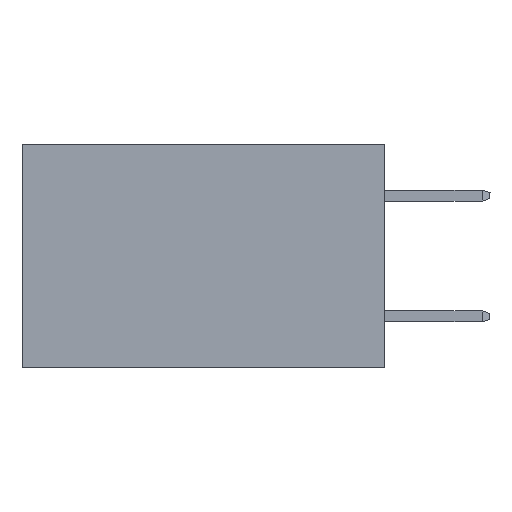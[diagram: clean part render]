
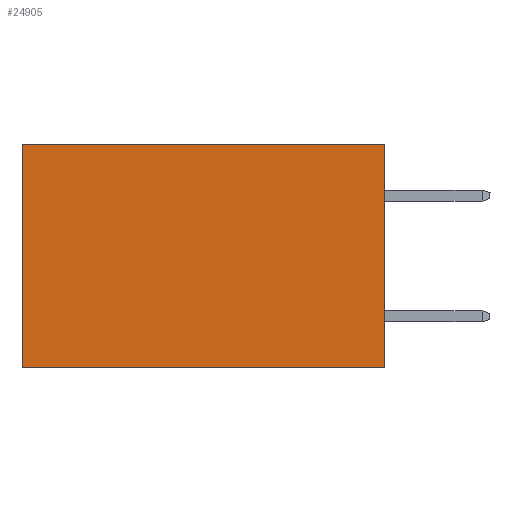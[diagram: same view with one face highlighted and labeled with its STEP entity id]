
A CAD part, left-side view. The second image highlights one B-rep face of the part: STEP entity #24905.
In plain terms, the highlighted planar face has unit normal (-1, 0, 0).
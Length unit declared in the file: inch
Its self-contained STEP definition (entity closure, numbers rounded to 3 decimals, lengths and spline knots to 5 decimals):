
#621 = ORIENTED_EDGE ( 'NONE', *, *, #26804, .F. ) ;
#1922 = DIRECTION ( 'NONE',  ( 0., 1., 0. ) ) ;
#1936 = VECTOR ( 'NONE', #1922, 39.37008 ) ;
#2787 = VERTEX_POINT ( 'NONE', #11318 ) ;
#4593 = CARTESIAN_POINT ( 'NONE',  ( 0.298, 0.6, 0. ) ) ;
#5815 = CARTESIAN_POINT ( 'NONE',  ( 0.298, 0., 0. ) ) ;
#6499 = LINE ( 'NONE', #24224, #23746 ) ;
#8424 = VECTOR ( 'NONE', #13081, 39.37008 ) ;
#10789 = ORIENTED_EDGE ( 'NONE', *, *, #15449, .T. ) ;
#10838 = DIRECTION ( 'NONE',  ( 0., 0., -1. ) ) ;
#11318 = CARTESIAN_POINT ( 'NONE',  ( 0.298, 0.6, -0.37 ) ) ;
#11441 = CARTESIAN_POINT ( 'NONE',  ( 0.298, 0., 0. ) ) ;
#13081 = DIRECTION ( 'NONE',  ( 0., 0., -1. ) ) ;
#15449 = EDGE_CURVE ( 'NONE', #24214, #26993, #22751, .T. ) ;
#16557 = EDGE_CURVE ( 'NONE', #24214, #19459, #6499, .T. ) ;
#17077 = DIRECTION ( 'NONE',  ( 1., 0., 0. ) ) ;
#17932 = AXIS2_PLACEMENT_3D ( 'NONE', #21419, #17077, #28034 ) ;
#18116 = FACE_OUTER_BOUND ( 'NONE', #19553, .T. ) ;
#19459 = VERTEX_POINT ( 'NONE', #22191 ) ;
#19553 = EDGE_LOOP ( 'NONE', ( #24367, #621, #21890, #10789 ) ) ;
#19876 = CARTESIAN_POINT ( 'NONE',  ( 0.298, 0.6, 0. ) ) ;
#21216 = PLANE ( 'NONE',  #17932 ) ;
#21419 = CARTESIAN_POINT ( 'NONE',  ( 0.298, 0., 0. ) ) ;
#21848 = EDGE_CURVE ( 'NONE', #26993, #2787, #26714, .T. ) ;
#21890 = ORIENTED_EDGE ( 'NONE', *, *, #16557, .F. ) ;
#22016 = LINE ( 'NONE', #26906, #1936 ) ;
#22191 = CARTESIAN_POINT ( 'NONE',  ( 0.298, 0., -0.37 ) ) ;
#22751 = LINE ( 'NONE', #11441, #23470 ) ;
#22754 = DIRECTION ( 'NONE',  ( 0., 1., 0. ) ) ;
#23470 = VECTOR ( 'NONE', #22754, 39.37008 ) ;
#23746 = VECTOR ( 'NONE', #10838, 39.37008 ) ;
#24214 = VERTEX_POINT ( 'NONE', #5815 ) ;
#24224 = CARTESIAN_POINT ( 'NONE',  ( 0.298, 0., 0. ) ) ;
#24367 = ORIENTED_EDGE ( 'NONE', *, *, #21848, .T. ) ;
#24905 = ADVANCED_FACE ( 'NONE', ( #18116 ), #21216, .F. ) ;
#26714 = LINE ( 'NONE', #19876, #8424 ) ;
#26804 = EDGE_CURVE ( 'NONE', #19459, #2787, #22016, .T. ) ;
#26906 = CARTESIAN_POINT ( 'NONE',  ( 0.298, 0., -0.37 ) ) ;
#26993 = VERTEX_POINT ( 'NONE', #4593 ) ;
#28034 = DIRECTION ( 'NONE',  ( 0., 0., -1. ) ) ;
